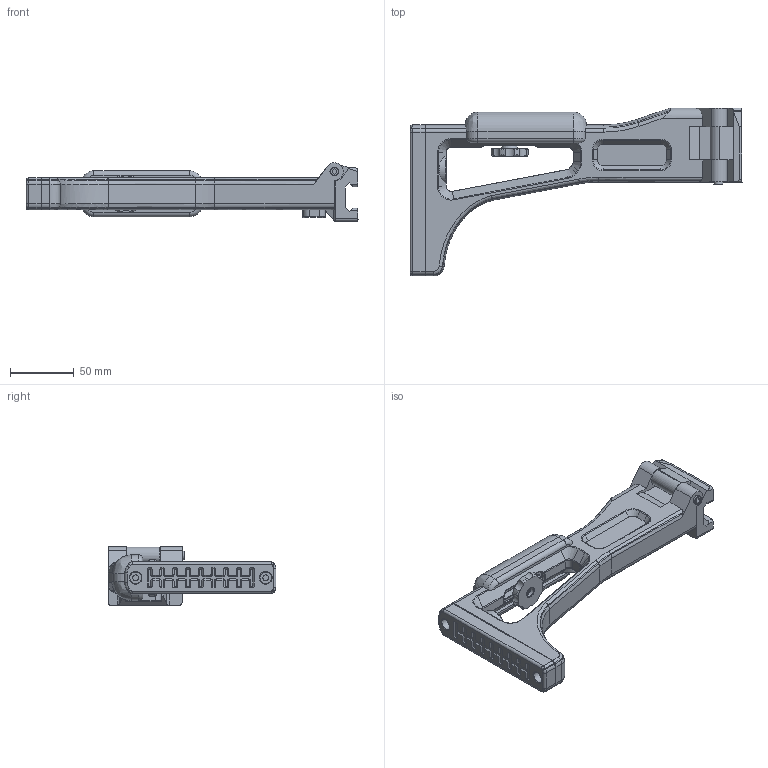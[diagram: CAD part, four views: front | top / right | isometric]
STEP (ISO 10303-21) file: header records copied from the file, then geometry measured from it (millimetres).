
FILE_DESCRIPTION(/* description */ (''),/* implementation_level */ '2;1');
FILE_NAME(/* name */ 'g36 stock hd.stp',/* time_stamp */ '2021-01-31T13:53:42+02:00',/* author */ (''),/* organization */ (''),/* preprocessor_version */ 'ST-DEVELOPER v15.2',/* originating_system */ 'Autodesk Translator Framework v2.0.0.5431',/* authorisation */ '');
FILE_SCHEMA (('AUTOMOTIVE_DESIGN { 1 0 10303 214 3 1 1 }'));
Length unit declared in the file: centimetre
Products named in the file (1): unpublished stocks2 G36 HD HINGE
Bounding box: 260.25 x 131.54 x 45.85 mm (x, y, z)
Volume: 349148.8 mm3; surface area: 87298.3 mm2
Topology: 7 solids, 7 shells, 739 faces, 1901 edges, 1190 vertices
Faces by surface type: plane 293, bspline 145, cone 133, cylinder 132, torus 36
Full cylindrical faces by diameter (mm): 3 x2, 3.6 x1, 4 x1, 4.2 x1, 4.5 x4, 4.6 x2, 5 x1, 7 x2, 8 x1, 9 x4, 9.6 x1, 10 x1
Entity records: 26819 total; most frequent: CARTESIAN_POINT 9444, ORIENTED_EDGE 3700, DIRECTION 3498, EDGE_CURVE 1850, AXIS2_PLACEMENT_3D 1244, VERTEX_POINT 1181, LINE 1010, VECTOR 1010
